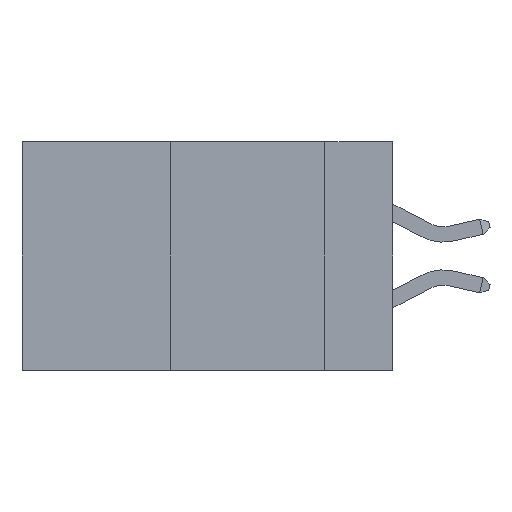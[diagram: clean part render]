
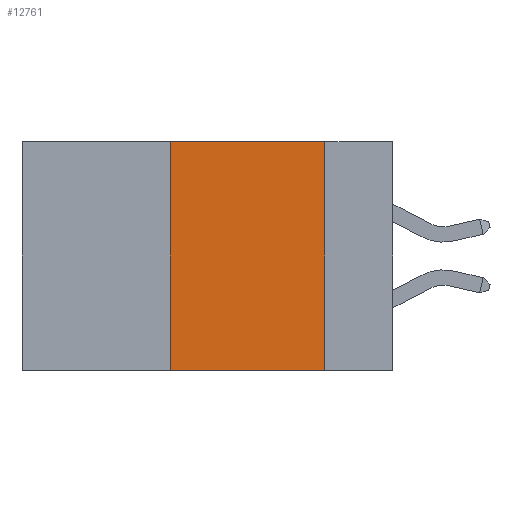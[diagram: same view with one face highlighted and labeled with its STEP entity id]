
A CAD part, left-side view. The second image highlights one B-rep face of the part: STEP entity #12761.
In plain terms, the highlighted planar face has unit normal (-1, 0, 0).
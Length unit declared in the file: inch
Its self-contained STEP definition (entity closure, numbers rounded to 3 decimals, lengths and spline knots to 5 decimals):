
#517 = ORIENTED_EDGE ( 'NONE', *, *, #10650, .F. ) ;
#2024 = LINE ( 'NONE', #3977, #11809 ) ;
#2495 = DIRECTION ( 'NONE',  ( 1., 0., 0. ) ) ;
#2499 = CARTESIAN_POINT ( 'NONE',  ( 0., 0.11, -0.37 ) ) ;
#2731 = DIRECTION ( 'NONE',  ( 0., 0., 1. ) ) ;
#2857 = CARTESIAN_POINT ( 'NONE',  ( 0., 0.11, 0. ) ) ;
#3569 = CARTESIAN_POINT ( 'NONE',  ( 0., 0.36, -0.37 ) ) ;
#3977 = CARTESIAN_POINT ( 'NONE',  ( 0., 0.6, 0. ) ) ;
#4425 = LINE ( 'NONE', #8717, #8202 ) ;
#4476 = PLANE ( 'NONE',  #12679 ) ;
#4716 = CARTESIAN_POINT ( 'NONE',  ( 0., 0.11, 0. ) ) ;
#4734 = DIRECTION ( 'NONE',  ( 0., -1., 0. ) ) ;
#5029 = VERTEX_POINT ( 'NONE', #3569 ) ;
#5144 = ORIENTED_EDGE ( 'NONE', *, *, #6120, .F. ) ;
#5171 = DIRECTION ( 'NONE',  ( 0., -1., 0. ) ) ;
#5497 = CARTESIAN_POINT ( 'NONE',  ( 0., 0.6, 0. ) ) ;
#5664 = VECTOR ( 'NONE', #10588, 39.37008 ) ;
#6120 = EDGE_CURVE ( 'NONE', #5029, #7356, #7601, .T. ) ;
#6636 = EDGE_CURVE ( 'NONE', #5029, #7633, #4425, .T. ) ;
#7356 = VERTEX_POINT ( 'NONE', #12936 ) ;
#7485 = DIRECTION ( 'NONE',  ( 0., 0., -1. ) ) ;
#7509 = FACE_OUTER_BOUND ( 'NONE', #12218, .T. ) ;
#7601 = LINE ( 'NONE', #12751, #10721 ) ;
#7633 = VERTEX_POINT ( 'NONE', #2499 ) ;
#8202 = VECTOR ( 'NONE', #4734, 39.37008 ) ;
#8717 = CARTESIAN_POINT ( 'NONE',  ( 0., 0.6, -0.37 ) ) ;
#10286 = ORIENTED_EDGE ( 'NONE', *, *, #6636, .T. ) ;
#10588 = DIRECTION ( 'NONE',  ( 0., 0., -1. ) ) ;
#10650 = EDGE_CURVE ( 'NONE', #12486, #7633, #11015, .T. ) ;
#10721 = VECTOR ( 'NONE', #2731, 39.37008 ) ;
#11015 = LINE ( 'NONE', #4716, #5664 ) ;
#11151 = EDGE_CURVE ( 'NONE', #7356, #12486, #2024, .T. ) ;
#11809 = VECTOR ( 'NONE', #5171, 39.37008 ) ;
#12218 = EDGE_LOOP ( 'NONE', ( #517, #12507, #5144, #10286 ) ) ;
#12486 = VERTEX_POINT ( 'NONE', #2857 ) ;
#12507 = ORIENTED_EDGE ( 'NONE', *, *, #11151, .F. ) ;
#12679 = AXIS2_PLACEMENT_3D ( 'NONE', #5497, #2495, #7485 ) ;
#12751 = CARTESIAN_POINT ( 'NONE',  ( 0., 0.36, 0. ) ) ;
#12761 = ADVANCED_FACE ( 'NONE', ( #7509 ), #4476, .F. ) ;
#12936 = CARTESIAN_POINT ( 'NONE',  ( 0., 0.36, 0. ) ) ;
